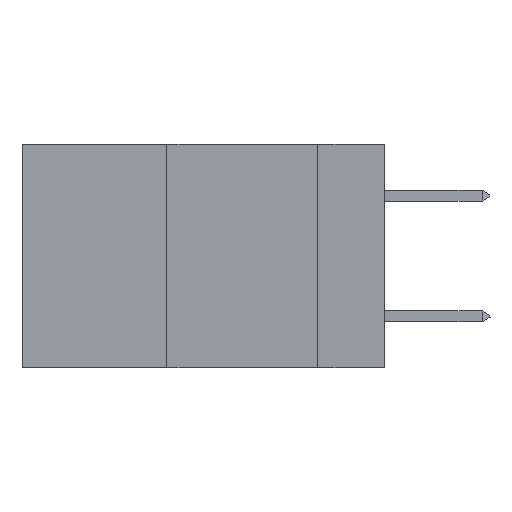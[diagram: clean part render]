
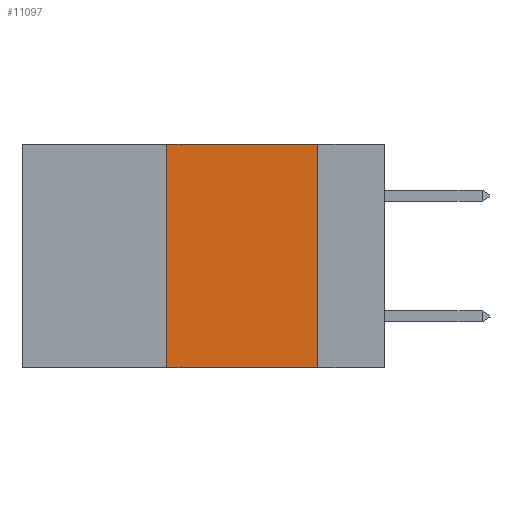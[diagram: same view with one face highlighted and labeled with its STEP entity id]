
A CAD part, left-side view. The second image highlights one B-rep face of the part: STEP entity #11097.
In plain terms, the highlighted planar face has unit normal (-1, 0, 0).
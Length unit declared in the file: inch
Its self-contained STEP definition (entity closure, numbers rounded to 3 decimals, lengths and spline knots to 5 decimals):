
#235 = LINE ( 'NONE', #13811, #18582 ) ;
#764 = VECTOR ( 'NONE', #6308, 39.37008 ) ;
#1152 = PLANE ( 'NONE',  #34837 ) ;
#1738 = CARTESIAN_POINT ( 'NONE',  ( 0., 0.36, 0. ) ) ;
#2581 = ORIENTED_EDGE ( 'NONE', *, *, #16846, .T. ) ;
#4334 = EDGE_CURVE ( 'NONE', #38660, #33194, #13188, .T. ) ;
#4604 = EDGE_CURVE ( 'NONE', #33194, #6739, #8167, .T. ) ;
#5361 = LINE ( 'NONE', #1738, #33992 ) ;
#6308 = DIRECTION ( 'NONE',  ( 0., 0., -1. ) ) ;
#6635 = DIRECTION ( 'NONE',  ( 0., -1., 0. ) ) ;
#6739 = VERTEX_POINT ( 'NONE', #27589 ) ;
#8167 = LINE ( 'NONE', #39639, #764 ) ;
#11097 = ADVANCED_FACE ( 'NONE', ( #11106 ), #1152, .F. ) ;
#11106 = FACE_OUTER_BOUND ( 'NONE', #42485, .T. ) ;
#11327 = DIRECTION ( 'NONE',  ( 1., 0., 0. ) ) ;
#13188 = LINE ( 'NONE', #33574, #42652 ) ;
#13811 = CARTESIAN_POINT ( 'NONE',  ( 0., 0.6, -0.37 ) ) ;
#14237 = DIRECTION ( 'NONE',  ( 0., -1., 0. ) ) ;
#15839 = CARTESIAN_POINT ( 'NONE',  ( 0., 0.11, 0. ) ) ;
#16846 = EDGE_CURVE ( 'NONE', #17143, #6739, #235, .T. ) ;
#17143 = VERTEX_POINT ( 'NONE', #23048 ) ;
#17571 = ORIENTED_EDGE ( 'NONE', *, *, #20101, .F. ) ;
#18582 = VECTOR ( 'NONE', #14237, 39.37008 ) ;
#20101 = EDGE_CURVE ( 'NONE', #17143, #38660, #5361, .T. ) ;
#23048 = CARTESIAN_POINT ( 'NONE',  ( 0., 0.36, -0.37 ) ) ;
#24919 = DIRECTION ( 'NONE',  ( 0., 0., -1. ) ) ;
#27589 = CARTESIAN_POINT ( 'NONE',  ( 0., 0.11, -0.37 ) ) ;
#28687 = DIRECTION ( 'NONE',  ( 0., 0., 1. ) ) ;
#31549 = ORIENTED_EDGE ( 'NONE', *, *, #4334, .F. ) ;
#33194 = VERTEX_POINT ( 'NONE', #15839 ) ;
#33574 = CARTESIAN_POINT ( 'NONE',  ( 0., 0.6, 0. ) ) ;
#33992 = VECTOR ( 'NONE', #28687, 39.37008 ) ;
#34837 = AXIS2_PLACEMENT_3D ( 'NONE', #35551, #11327, #24919 ) ;
#35551 = CARTESIAN_POINT ( 'NONE',  ( 0., 0.6, 0. ) ) ;
#38660 = VERTEX_POINT ( 'NONE', #43864 ) ;
#39639 = CARTESIAN_POINT ( 'NONE',  ( 0., 0.11, 0. ) ) ;
#42485 = EDGE_LOOP ( 'NONE', ( #43150, #31549, #17571, #2581 ) ) ;
#42652 = VECTOR ( 'NONE', #6635, 39.37008 ) ;
#43150 = ORIENTED_EDGE ( 'NONE', *, *, #4604, .F. ) ;
#43864 = CARTESIAN_POINT ( 'NONE',  ( 0., 0.36, 0. ) ) ;
